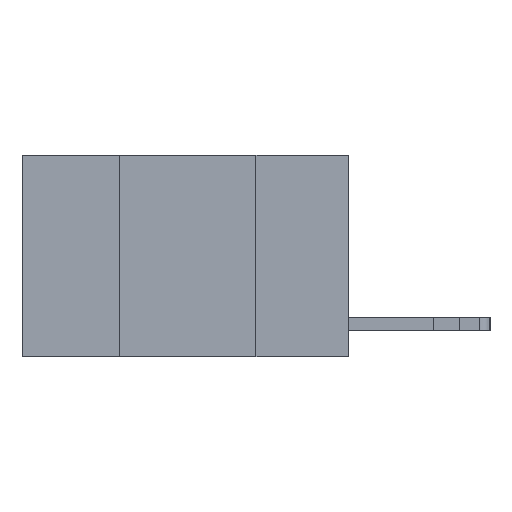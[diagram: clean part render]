
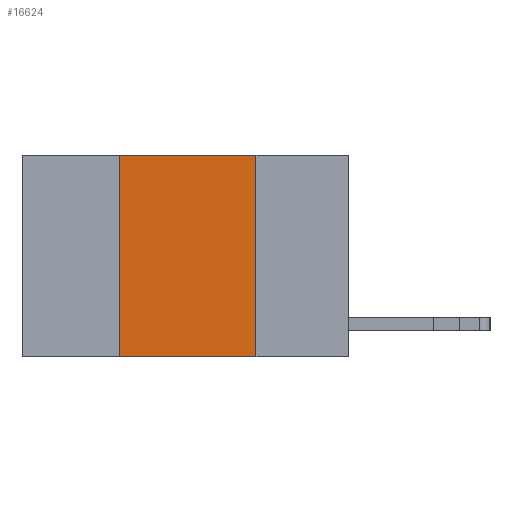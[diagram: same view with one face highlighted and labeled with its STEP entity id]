
A CAD part, left-side view. The second image highlights one B-rep face of the part: STEP entity #16624.
In plain terms, the highlighted planar face has unit normal (-1, 0, 0).
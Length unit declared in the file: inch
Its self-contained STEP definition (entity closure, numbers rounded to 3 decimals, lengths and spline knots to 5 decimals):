
#738 = VERTEX_POINT ( 'NONE', #9265 ) ;
#1340 = DIRECTION ( 'NONE',  ( 1., 0., 0. ) ) ;
#2405 = CARTESIAN_POINT ( 'NONE',  ( 0., 0.6, 0. ) ) ;
#3094 = DIRECTION ( 'NONE',  ( 0., 0., -1. ) ) ;
#4047 = CARTESIAN_POINT ( 'NONE',  ( 0., 0.17, -0.37 ) ) ;
#4339 = DIRECTION ( 'NONE',  ( 0., -1., 0. ) ) ;
#4545 = EDGE_CURVE ( 'NONE', #738, #21682, #20686, .T. ) ;
#6112 = VECTOR ( 'NONE', #16734, 39.37008 ) ;
#6734 = FACE_OUTER_BOUND ( 'NONE', #13504, .T. ) ;
#7704 = CARTESIAN_POINT ( 'NONE',  ( 0., 0.42, -0.37 ) ) ;
#7837 = ORIENTED_EDGE ( 'NONE', *, *, #22686, .F. ) ;
#7995 = CARTESIAN_POINT ( 'NONE',  ( 0., 0.17, 0. ) ) ;
#8352 = CARTESIAN_POINT ( 'NONE',  ( 0., 0.42, 0. ) ) ;
#8588 = LINE ( 'NONE', #8352, #18520 ) ;
#8801 = ORIENTED_EDGE ( 'NONE', *, *, #4545, .F. ) ;
#8860 = VERTEX_POINT ( 'NONE', #7704 ) ;
#9265 = CARTESIAN_POINT ( 'NONE',  ( 0., 0.42, 0. ) ) ;
#9597 = VECTOR ( 'NONE', #4339, 39.37008 ) ;
#9765 = LINE ( 'NONE', #7995, #9920 ) ;
#9920 = VECTOR ( 'NONE', #15069, 39.37008 ) ;
#10033 = PLANE ( 'NONE',  #18801 ) ;
#12061 = ORIENTED_EDGE ( 'NONE', *, *, #23037, .F. ) ;
#13504 = EDGE_LOOP ( 'NONE', ( #12061, #8801, #7837, #15712 ) ) ;
#14024 = CARTESIAN_POINT ( 'NONE',  ( 0., 0.6, 0. ) ) ;
#15069 = DIRECTION ( 'NONE',  ( 0., 0., -1. ) ) ;
#15712 = ORIENTED_EDGE ( 'NONE', *, *, #18701, .T. ) ;
#16479 = CARTESIAN_POINT ( 'NONE',  ( 0., 0.17, 0. ) ) ;
#16624 = ADVANCED_FACE ( 'NONE', ( #6734 ), #10033, .F. ) ;
#16734 = DIRECTION ( 'NONE',  ( 0., -1., 0. ) ) ;
#17163 = CARTESIAN_POINT ( 'NONE',  ( 0., 0.6, -0.37 ) ) ;
#17663 = DIRECTION ( 'NONE',  ( 0., 0., 1. ) ) ;
#18520 = VECTOR ( 'NONE', #17663, 39.37008 ) ;
#18701 = EDGE_CURVE ( 'NONE', #8860, #22450, #20762, .T. ) ;
#18801 = AXIS2_PLACEMENT_3D ( 'NONE', #14024, #1340, #3094 ) ;
#20686 = LINE ( 'NONE', #2405, #6112 ) ;
#20762 = LINE ( 'NONE', #17163, #9597 ) ;
#21682 = VERTEX_POINT ( 'NONE', #16479 ) ;
#22450 = VERTEX_POINT ( 'NONE', #4047 ) ;
#22686 = EDGE_CURVE ( 'NONE', #8860, #738, #8588, .T. ) ;
#23037 = EDGE_CURVE ( 'NONE', #21682, #22450, #9765, .T. ) ;
